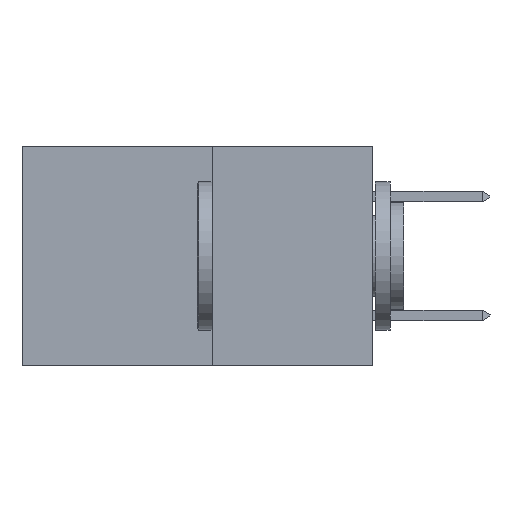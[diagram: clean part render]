
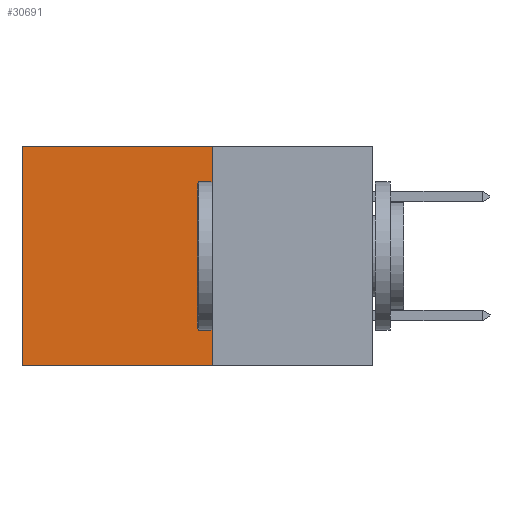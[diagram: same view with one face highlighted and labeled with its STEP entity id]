
A CAD part, left-side view. The second image highlights one B-rep face of the part: STEP entity #30691.
In plain terms, the highlighted planar face has unit normal (-1, 0, 0).
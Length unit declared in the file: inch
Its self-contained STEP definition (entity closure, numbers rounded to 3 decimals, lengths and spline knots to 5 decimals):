
#230 = DIRECTION ( 'NONE',  ( 0., 1., 0. ) ) ;
#514 = CARTESIAN_POINT ( 'NONE',  ( 0.277, 0.27, -0.37 ) ) ;
#960 = VERTEX_POINT ( 'NONE', #13697 ) ;
#1041 = ORIENTED_EDGE ( 'NONE', *, *, #17302, .T. ) ;
#2264 = VECTOR ( 'NONE', #32412, 39.37008 ) ;
#2817 = EDGE_CURVE ( 'NONE', #960, #20297, #11479, .T. ) ;
#3840 = PLANE ( 'NONE',  #27156 ) ;
#4311 = VERTEX_POINT ( 'NONE', #23600 ) ;
#5685 = EDGE_CURVE ( 'NONE', #4311, #15131, #34708, .T. ) ;
#5822 = VECTOR ( 'NONE', #27642, 39.37008 ) ;
#8803 = LINE ( 'NONE', #29635, #2264 ) ;
#11479 = LINE ( 'NONE', #31432, #13215 ) ;
#12216 = FACE_OUTER_BOUND ( 'NONE', #26033, .T. ) ;
#12234 = CARTESIAN_POINT ( 'NONE',  ( 0.277, 0.27, -0.37 ) ) ;
#13215 = VECTOR ( 'NONE', #30701, 39.37008 ) ;
#13697 = CARTESIAN_POINT ( 'NONE',  ( 0.277, 0.27, 0. ) ) ;
#15055 = DIRECTION ( 'NONE',  ( 0., 0., -1. ) ) ;
#15131 = VERTEX_POINT ( 'NONE', #21411 ) ;
#17302 = EDGE_CURVE ( 'NONE', #20297, #15131, #8803, .T. ) ;
#20297 = VERTEX_POINT ( 'NONE', #20959 ) ;
#20959 = CARTESIAN_POINT ( 'NONE',  ( 0.277, 0.59, 0. ) ) ;
#21411 = CARTESIAN_POINT ( 'NONE',  ( 0.277, 0.59, -0.37 ) ) ;
#23600 = CARTESIAN_POINT ( 'NONE',  ( 0.277, 0.27, -0.37 ) ) ;
#26033 = EDGE_LOOP ( 'NONE', ( #1041, #33917, #34882, #26390 ) ) ;
#26390 = ORIENTED_EDGE ( 'NONE', *, *, #2817, .T. ) ;
#27156 = AXIS2_PLACEMENT_3D ( 'NONE', #12234, #31684, #15055 ) ;
#27218 = LINE ( 'NONE', #35864, #5822 ) ;
#27413 = VECTOR ( 'NONE', #230, 39.37008 ) ;
#27642 = DIRECTION ( 'NONE',  ( 0., 0., -1. ) ) ;
#29635 = CARTESIAN_POINT ( 'NONE',  ( 0.277, 0.59, -0.37 ) ) ;
#30691 = ADVANCED_FACE ( 'NONE', ( #12216 ), #3840, .F. ) ;
#30701 = DIRECTION ( 'NONE',  ( 0., 1., 0. ) ) ;
#31432 = CARTESIAN_POINT ( 'NONE',  ( 0.277, 0.27, 0. ) ) ;
#31684 = DIRECTION ( 'NONE',  ( 1., 0., 0. ) ) ;
#32412 = DIRECTION ( 'NONE',  ( 0., 0., -1. ) ) ;
#33712 = EDGE_CURVE ( 'NONE', #960, #4311, #27218, .T. ) ;
#33917 = ORIENTED_EDGE ( 'NONE', *, *, #5685, .F. ) ;
#34708 = LINE ( 'NONE', #514, #27413 ) ;
#34882 = ORIENTED_EDGE ( 'NONE', *, *, #33712, .F. ) ;
#35864 = CARTESIAN_POINT ( 'NONE',  ( 0.277, 0.27, -0.37 ) ) ;
